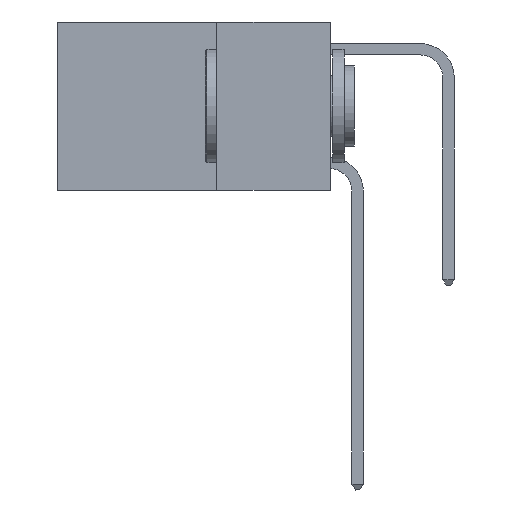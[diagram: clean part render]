
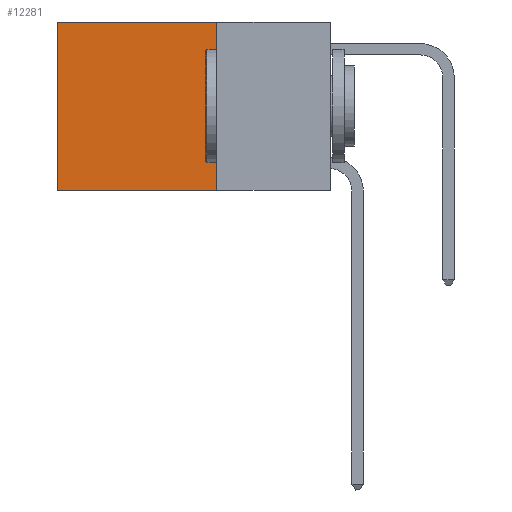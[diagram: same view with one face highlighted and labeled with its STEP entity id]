
A CAD part, left-side view. The second image highlights one B-rep face of the part: STEP entity #12281.
In plain terms, the highlighted planar face has unit normal (-1, 0, 0).
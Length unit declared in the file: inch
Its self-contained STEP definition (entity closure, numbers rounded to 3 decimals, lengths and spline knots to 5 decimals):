
#80 = PLANE ( 'NONE',  #8869 ) ;
#896 = EDGE_LOOP ( 'NONE', ( #6693, #9192, #18645, #11751 ) ) ;
#1646 = DIRECTION ( 'NONE',  ( 0., 1., 0. ) ) ;
#2119 = VECTOR ( 'NONE', #16456, 39.37008 ) ;
#2586 = VERTEX_POINT ( 'NONE', #5276 ) ;
#2711 = LINE ( 'NONE', #4883, #3205 ) ;
#3205 = VECTOR ( 'NONE', #15369, 39.37008 ) ;
#3286 = EDGE_CURVE ( 'NONE', #2586, #16898, #18508, .T. ) ;
#4766 = DIRECTION ( 'NONE',  ( 0., 0., -1. ) ) ;
#4859 = CARTESIAN_POINT ( 'NONE',  ( 0.2625, 0.6, 0. ) ) ;
#4883 = CARTESIAN_POINT ( 'NONE',  ( 0.2625, 0.6, 0. ) ) ;
#5276 = CARTESIAN_POINT ( 'NONE',  ( 0.2625, 0.25, -0.37 ) ) ;
#5544 = VECTOR ( 'NONE', #4766, 39.37008 ) ;
#6111 = VECTOR ( 'NONE', #1646, 39.37008 ) ;
#6375 = DIRECTION ( 'NONE',  ( 1., 0., 0. ) ) ;
#6693 = ORIENTED_EDGE ( 'NONE', *, *, #7968, .T. ) ;
#7968 = EDGE_CURVE ( 'NONE', #13529, #16898, #2711, .T. ) ;
#8869 = AXIS2_PLACEMENT_3D ( 'NONE', #15316, #6375, #16776 ) ;
#9024 = CARTESIAN_POINT ( 'NONE',  ( 0.2625, 0.25, -0.37 ) ) ;
#9192 = ORIENTED_EDGE ( 'NONE', *, *, #3286, .F. ) ;
#9297 = CARTESIAN_POINT ( 'NONE',  ( 0.2625, 0.25, 0. ) ) ;
#11751 = ORIENTED_EDGE ( 'NONE', *, *, #15921, .T. ) ;
#12281 = ADVANCED_FACE ( 'NONE', ( #15501 ), #80, .F. ) ;
#13529 = VERTEX_POINT ( 'NONE', #4859 ) ;
#13588 = LINE ( 'NONE', #13886, #5544 ) ;
#13886 = CARTESIAN_POINT ( 'NONE',  ( 0.2625, 0.25, 0. ) ) ;
#14672 = VERTEX_POINT ( 'NONE', #17655 ) ;
#14789 = CARTESIAN_POINT ( 'NONE',  ( 0.2625, 0.6, -0.37 ) ) ;
#15316 = CARTESIAN_POINT ( 'NONE',  ( 0.2625, 0.25, 0. ) ) ;
#15369 = DIRECTION ( 'NONE',  ( 0., 0., -1. ) ) ;
#15501 = FACE_OUTER_BOUND ( 'NONE', #896, .T. ) ;
#15921 = EDGE_CURVE ( 'NONE', #14672, #13529, #17945, .T. ) ;
#16456 = DIRECTION ( 'NONE',  ( 0., 1., 0. ) ) ;
#16776 = DIRECTION ( 'NONE',  ( 0., 0., -1. ) ) ;
#16898 = VERTEX_POINT ( 'NONE', #14789 ) ;
#17655 = CARTESIAN_POINT ( 'NONE',  ( 0.2625, 0.25, 0. ) ) ;
#17741 = EDGE_CURVE ( 'NONE', #14672, #2586, #13588, .T. ) ;
#17945 = LINE ( 'NONE', #9297, #6111 ) ;
#18508 = LINE ( 'NONE', #9024, #2119 ) ;
#18645 = ORIENTED_EDGE ( 'NONE', *, *, #17741, .F. ) ;
